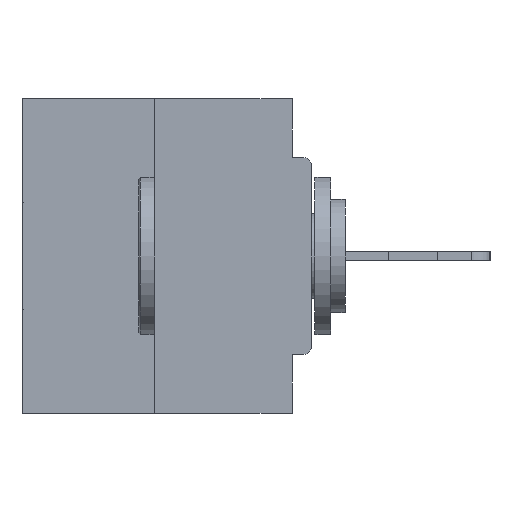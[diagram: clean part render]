
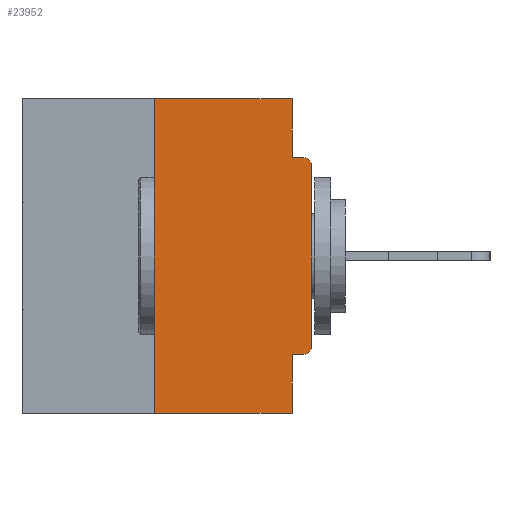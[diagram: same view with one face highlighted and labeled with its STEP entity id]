
A CAD part, left-side view. The second image highlights one B-rep face of the part: STEP entity #23952.
In plain terms, the highlighted planar face has unit normal (-1, 0, 0).
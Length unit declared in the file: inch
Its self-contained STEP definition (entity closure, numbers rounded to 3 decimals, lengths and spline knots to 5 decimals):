
#101 = VERTEX_POINT ( 'NONE', #16379 ) ;
#397 = CARTESIAN_POINT ( 'NONE',  ( 0., 0., -0.0935 ) ) ;
#982 = EDGE_CURVE ( 'NONE', #11802, #27183, #30600, .T. ) ;
#1440 = CARTESIAN_POINT ( 'NONE',  ( 0., 0.46, 0. ) ) ;
#1939 = VERTEX_POINT ( 'NONE', #14358 ) ;
#2225 = DIRECTION ( 'NONE',  ( 0., 0., -1. ) ) ;
#2528 = DIRECTION ( 'NONE',  ( 0., -1., 0. ) ) ;
#3168 = DIRECTION ( 'NONE',  ( 0., -1., 0. ) ) ;
#3652 = VERTEX_POINT ( 'NONE', #17387 ) ;
#3992 = VECTOR ( 'NONE', #20088, 39.37008 ) ;
#4239 = VERTEX_POINT ( 'NONE', #12480 ) ;
#4411 = CARTESIAN_POINT ( 'NONE',  ( 0., 0.015, -0.1085 ) ) ;
#5095 = CARTESIAN_POINT ( 'NONE',  ( 0., 0.015, -0.4065 ) ) ;
#5215 = CARTESIAN_POINT ( 'NONE',  ( 0., 0.46, -0.5 ) ) ;
#5361 = CARTESIAN_POINT ( 'NONE',  ( 0., 0.031, -0.5 ) ) ;
#5622 = LINE ( 'NONE', #12629, #32523 ) ;
#5992 = LINE ( 'NONE', #397, #32071 ) ;
#6360 = AXIS2_PLACEMENT_3D ( 'NONE', #30954, #18125, #2225 ) ;
#7124 = DIRECTION ( 'NONE',  ( 0., 0., -1. ) ) ;
#7478 = CARTESIAN_POINT ( 'NONE',  ( 0., 0.015, -0.3915 ) ) ;
#7945 = CARTESIAN_POINT ( 'NONE',  ( 0., 0.25, 0. ) ) ;
#9364 = ORIENTED_EDGE ( 'NONE', *, *, #19771, .F. ) ;
#9452 = EDGE_CURVE ( 'NONE', #1939, #3652, #23008, .T. ) ;
#9751 = VERTEX_POINT ( 'NONE', #17152 ) ;
#10151 = DIRECTION ( 'NONE',  ( 0., 0., -1. ) ) ;
#10426 = EDGE_CURVE ( 'NONE', #31745, #9751, #5622, .T. ) ;
#10715 = LINE ( 'NONE', #5215, #16887 ) ;
#10790 = VECTOR ( 'NONE', #21402, 39.37008 ) ;
#11802 = VERTEX_POINT ( 'NONE', #29075 ) ;
#12480 = CARTESIAN_POINT ( 'NONE',  ( 0., 0.031, -0.4065 ) ) ;
#12629 = CARTESIAN_POINT ( 'NONE',  ( 0., 0.031, 0. ) ) ;
#12774 = LINE ( 'NONE', #25173, #3992 ) ;
#12875 = ORIENTED_EDGE ( 'NONE', *, *, #10426, .F. ) ;
#13744 = VECTOR ( 'NONE', #27788, 39.37008 ) ;
#14076 = DIRECTION ( 'NONE',  ( 0., 0., 1. ) ) ;
#14358 = CARTESIAN_POINT ( 'NONE',  ( 0., 0.25, -0.5 ) ) ;
#15454 = FACE_OUTER_BOUND ( 'NONE', #17990, .T. ) ;
#15528 = PLANE ( 'NONE',  #6360 ) ;
#16109 = VECTOR ( 'NONE', #21038, 39.37008 ) ;
#16379 = CARTESIAN_POINT ( 'NONE',  ( 0., 0.015, -0.0935 ) ) ;
#16887 = VECTOR ( 'NONE', #2528, 39.37008 ) ;
#16962 = CARTESIAN_POINT ( 'NONE',  ( 0., 0., 0. ) ) ;
#17152 = CARTESIAN_POINT ( 'NONE',  ( 0., 0.031, -0.0935 ) ) ;
#17312 = CIRCLE ( 'NONE', #33365, 0.015 ) ;
#17387 = CARTESIAN_POINT ( 'NONE',  ( 0., 0.25, 0. ) ) ;
#17921 = CARTESIAN_POINT ( 'NONE',  ( 0., 0.031, 0. ) ) ;
#17990 = EDGE_LOOP ( 'NONE', ( #9364, #22877, #20480, #26122, #30936, #28195, #23789, #31773, #31061, #12875 ) ) ;
#18125 = DIRECTION ( 'NONE',  ( 1., 0., 0. ) ) ;
#19771 = EDGE_CURVE ( 'NONE', #3652, #31745, #20695, .T. ) ;
#20088 = DIRECTION ( 'NONE',  ( 0., 1., 0. ) ) ;
#20480 = ORIENTED_EDGE ( 'NONE', *, *, #33346, .T. ) ;
#20695 = LINE ( 'NONE', #1440, #13744 ) ;
#21038 = DIRECTION ( 'NONE',  ( 0., 0., 1. ) ) ;
#21123 = CIRCLE ( 'NONE', #30974, 0.015 ) ;
#21402 = DIRECTION ( 'NONE',  ( 0., 0., -1. ) ) ;
#22036 = EDGE_CURVE ( 'NONE', #33313, #4239, #12774, .T. ) ;
#22860 = DIRECTION ( 'NONE',  ( -1., 0., 0. ) ) ;
#22877 = ORIENTED_EDGE ( 'NONE', *, *, #9452, .F. ) ;
#22914 = CARTESIAN_POINT ( 'NONE',  ( 0., 0.031, -0.5 ) ) ;
#22981 = VECTOR ( 'NONE', #14076, 39.37008 ) ;
#23008 = LINE ( 'NONE', #7945, #16109 ) ;
#23789 = ORIENTED_EDGE ( 'NONE', *, *, #982, .T. ) ;
#23855 = VERTEX_POINT ( 'NONE', #22914 ) ;
#23952 = ADVANCED_FACE ( 'NONE', ( #15454 ), #15528, .F. ) ;
#25173 = CARTESIAN_POINT ( 'NONE',  ( 0., 0., -0.4065 ) ) ;
#25766 = DIRECTION ( 'NONE',  ( -1., 0., 0. ) ) ;
#26122 = ORIENTED_EDGE ( 'NONE', *, *, #32468, .F. ) ;
#27183 = VERTEX_POINT ( 'NONE', #29422 ) ;
#27788 = DIRECTION ( 'NONE',  ( 0., -1., 0. ) ) ;
#28195 = ORIENTED_EDGE ( 'NONE', *, *, #31116, .T. ) ;
#28244 = EDGE_CURVE ( 'NONE', #9751, #101, #5992, .T. ) ;
#29075 = CARTESIAN_POINT ( 'NONE',  ( 0., 0., -0.3915 ) ) ;
#29422 = CARTESIAN_POINT ( 'NONE',  ( 0., 0., -0.1085 ) ) ;
#30600 = LINE ( 'NONE', #16962, #22981 ) ;
#30730 = DIRECTION ( 'NONE',  ( 0., 0., -1. ) ) ;
#30936 = ORIENTED_EDGE ( 'NONE', *, *, #22036, .F. ) ;
#30954 = CARTESIAN_POINT ( 'NONE',  ( 0., 0.46, 0. ) ) ;
#30974 = AXIS2_PLACEMENT_3D ( 'NONE', #7478, #25766, #10151 ) ;
#31061 = ORIENTED_EDGE ( 'NONE', *, *, #28244, .F. ) ;
#31116 = EDGE_CURVE ( 'NONE', #33313, #11802, #21123, .T. ) ;
#31433 = LINE ( 'NONE', #5361, #10790 ) ;
#31745 = VERTEX_POINT ( 'NONE', #17921 ) ;
#31773 = ORIENTED_EDGE ( 'NONE', *, *, #33149, .T. ) ;
#32071 = VECTOR ( 'NONE', #3168, 39.37008 ) ;
#32468 = EDGE_CURVE ( 'NONE', #4239, #23855, #31433, .T. ) ;
#32523 = VECTOR ( 'NONE', #30730, 39.37008 ) ;
#33149 = EDGE_CURVE ( 'NONE', #27183, #101, #17312, .T. ) ;
#33313 = VERTEX_POINT ( 'NONE', #5095 ) ;
#33346 = EDGE_CURVE ( 'NONE', #1939, #23855, #10715, .T. ) ;
#33365 = AXIS2_PLACEMENT_3D ( 'NONE', #4411, #22860, #7124 ) ;
